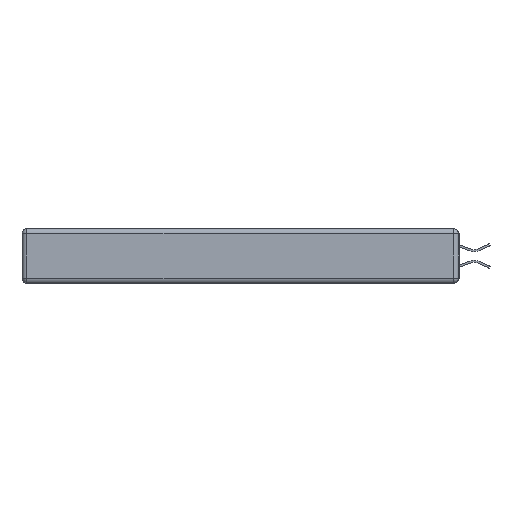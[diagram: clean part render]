
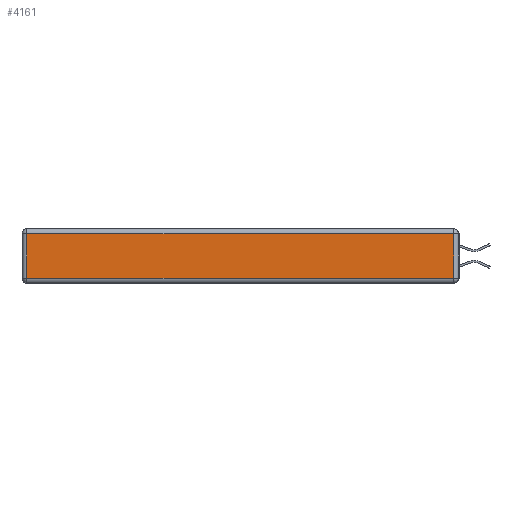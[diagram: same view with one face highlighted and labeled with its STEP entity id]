
A CAD part, left-side view. The second image highlights one B-rep face of the part: STEP entity #4161.
In plain terms, the highlighted planar face has unit normal (-1, 0, 0).
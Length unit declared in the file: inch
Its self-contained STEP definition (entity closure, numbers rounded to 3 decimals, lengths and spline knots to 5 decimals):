
#68 = CARTESIAN_POINT ( 'NONE',  ( 0., 2.75, -0.03 ) ) ;
#159 = EDGE_CURVE ( 'NONE', #11768, #9942, #16724, .T. ) ;
#732 = VECTOR ( 'NONE', #9042, 39.37008 ) ;
#948 = LINE ( 'NONE', #68, #732 ) ;
#1289 = EDGE_LOOP ( 'NONE', ( #7081, #3736, #13851, #15501 ) ) ;
#1701 = DIRECTION ( 'NONE',  ( 0., 0., 1. ) ) ;
#1917 = VECTOR ( 'NONE', #15963, 39.37008 ) ;
#3218 = VECTOR ( 'NONE', #11939, 39.37008 ) ;
#3736 = ORIENTED_EDGE ( 'NONE', *, *, #13459, .T. ) ;
#3977 = CARTESIAN_POINT ( 'NONE',  ( 0., 2.72, -0.343 ) ) ;
#4161 = ADVANCED_FACE ( 'NONE', ( #10119 ), #5620, .T. ) ;
#4318 = CARTESIAN_POINT ( 'NONE',  ( 0., 2.72, -0.313 ) ) ;
#4621 = LINE ( 'NONE', #11801, #7507 ) ;
#5620 = PLANE ( 'NONE',  #12022 ) ;
#5629 = CARTESIAN_POINT ( 'NONE',  ( 0., 0., -0.313 ) ) ;
#5677 = CARTESIAN_POINT ( 'NONE',  ( 0., 0., -0.343 ) ) ;
#6985 = DIRECTION ( 'NONE',  ( 0., 0., 1. ) ) ;
#7081 = ORIENTED_EDGE ( 'NONE', *, *, #159, .T. ) ;
#7507 = VECTOR ( 'NONE', #1701, 39.37008 ) ;
#7558 = CARTESIAN_POINT ( 'NONE',  ( 0., 0.03, -0.03 ) ) ;
#8691 = EDGE_CURVE ( 'NONE', #13127, #11768, #8747, .T. ) ;
#8747 = LINE ( 'NONE', #3977, #3218 ) ;
#9042 = DIRECTION ( 'NONE',  ( 0., 1., 0. ) ) ;
#9942 = VERTEX_POINT ( 'NONE', #10318 ) ;
#10119 = FACE_OUTER_BOUND ( 'NONE', #1289, .T. ) ;
#10318 = CARTESIAN_POINT ( 'NONE',  ( 0., 0.03, -0.313 ) ) ;
#10789 = DIRECTION ( 'NONE',  ( -1., 0., 0. ) ) ;
#11768 = VERTEX_POINT ( 'NONE', #4318 ) ;
#11801 = CARTESIAN_POINT ( 'NONE',  ( 0., 0.03, -0.343 ) ) ;
#11822 = CARTESIAN_POINT ( 'NONE',  ( 0., 2.72, -0.03 ) ) ;
#11939 = DIRECTION ( 'NONE',  ( 0., 0., -1. ) ) ;
#12022 = AXIS2_PLACEMENT_3D ( 'NONE', #5677, #10789, #6985 ) ;
#12150 = VERTEX_POINT ( 'NONE', #7558 ) ;
#13127 = VERTEX_POINT ( 'NONE', #11822 ) ;
#13459 = EDGE_CURVE ( 'NONE', #9942, #12150, #4621, .T. ) ;
#13851 = ORIENTED_EDGE ( 'NONE', *, *, #14685, .T. ) ;
#14685 = EDGE_CURVE ( 'NONE', #12150, #13127, #948, .T. ) ;
#15501 = ORIENTED_EDGE ( 'NONE', *, *, #8691, .T. ) ;
#15963 = DIRECTION ( 'NONE',  ( 0., -1., 0. ) ) ;
#16724 = LINE ( 'NONE', #5629, #1917 ) ;
